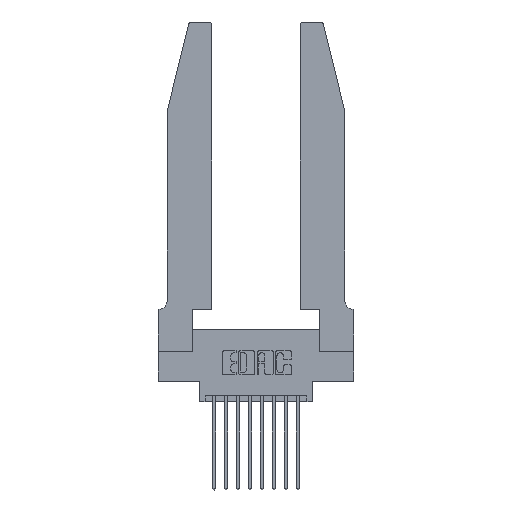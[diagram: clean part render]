
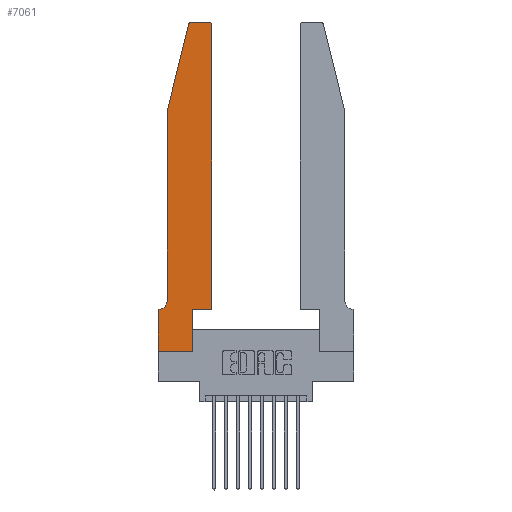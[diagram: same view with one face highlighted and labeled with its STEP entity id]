
A CAD part, top view. The second image highlights one B-rep face of the part: STEP entity #7061.
In plain terms, the highlighted planar face has unit normal (0, 0, 1).
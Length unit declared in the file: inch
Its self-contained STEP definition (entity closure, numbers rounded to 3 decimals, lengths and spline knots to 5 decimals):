
#55 = DIRECTION ( 'NONE',  ( 0., 1., 0. ) ) ;
#115 = VERTEX_POINT ( 'NONE', #11063 ) ;
#137 = VECTOR ( 'NONE', #9195, 39.37008 ) ;
#237 = LINE ( 'NONE', #2877, #425 ) ;
#254 = VERTEX_POINT ( 'NONE', #6310 ) ;
#397 = DIRECTION ( 'NONE',  ( 1., 0., 0. ) ) ;
#425 = VECTOR ( 'NONE', #13838, 39.37008 ) ;
#460 = VECTOR ( 'NONE', #7945, 39.37008 ) ;
#1157 = EDGE_CURVE ( 'NONE', #11795, #1531, #6339, .T. ) ;
#1382 = AXIS2_PLACEMENT_3D ( 'NONE', #1407, #3936, #6292 ) ;
#1407 = CARTESIAN_POINT ( 'NONE',  ( 0.0055, 0.42, 0.37 ) ) ;
#1531 = VERTEX_POINT ( 'NONE', #13340 ) ;
#1560 = DIRECTION ( 'NONE',  ( 0., 0., 1. ) ) ;
#1783 = LINE ( 'NONE', #11707, #460 ) ;
#1926 = CARTESIAN_POINT ( 'NONE',  ( 0.0755, 2., 0.37 ) ) ;
#2035 = CIRCLE ( 'NONE', #1382, 0.07 ) ;
#2506 = ORIENTED_EDGE ( 'NONE', *, *, #3610, .T. ) ;
#2720 = LINE ( 'NONE', #12124, #10547 ) ;
#2877 = CARTESIAN_POINT ( 'NONE',  ( 0.4505, 0.35, 0.37 ) ) ;
#3466 = LINE ( 'NONE', #9100, #14325 ) ;
#3610 = EDGE_CURVE ( 'NONE', #4110, #3991, #11367, .T. ) ;
#3641 = DIRECTION ( 'NONE',  ( 0., 1., 0. ) ) ;
#3936 = DIRECTION ( 'NONE',  ( 0., 0., -1. ) ) ;
#3991 = VERTEX_POINT ( 'NONE', #4832 ) ;
#4051 = VERTEX_POINT ( 'NONE', #15708 ) ;
#4110 = VERTEX_POINT ( 'NONE', #13651 ) ;
#4287 = ORIENTED_EDGE ( 'NONE', *, *, #9130, .T. ) ;
#4391 = LINE ( 'NONE', #13379, #8354 ) ;
#4583 = CARTESIAN_POINT ( 'NONE',  ( 0.4505, 0.35, 0.37 ) ) ;
#4595 = CARTESIAN_POINT ( 'NONE',  ( 0.0755, 2., 0.37 ) ) ;
#4832 = CARTESIAN_POINT ( 'NONE',  ( 0., 0., 0.37 ) ) ;
#4838 = ORIENTED_EDGE ( 'NONE', *, *, #13740, .T. ) ;
#5462 = VERTEX_POINT ( 'NONE', #14276 ) ;
#5578 = CARTESIAN_POINT ( 'NONE',  ( 0.25487, 2.72718, 0.37 ) ) ;
#5922 = VERTEX_POINT ( 'NONE', #12003 ) ;
#6208 = ORIENTED_EDGE ( 'NONE', *, *, #11518, .T. ) ;
#6292 = DIRECTION ( 'NONE',  ( -1., 0., 0. ) ) ;
#6310 = CARTESIAN_POINT ( 'NONE',  ( 0.2865, 0., 0.37 ) ) ;
#6339 = CIRCLE ( 'NONE', #13452, 0.03 ) ;
#6708 = CARTESIAN_POINT ( 'NONE',  ( 0.4505, 2.72, 0.37 ) ) ;
#7061 = ADVANCED_FACE ( 'NONE', ( #10238 ), #12466, .T. ) ;
#7253 = VERTEX_POINT ( 'NONE', #5578 ) ;
#7313 = LINE ( 'NONE', #4595, #12444 ) ;
#7570 = EDGE_CURVE ( 'NONE', #4051, #5922, #2035, .T. ) ;
#7691 = DIRECTION ( 'NONE',  ( 1., 0., 0. ) ) ;
#7941 = CARTESIAN_POINT ( 'NONE',  ( 0., 0., 0.37 ) ) ;
#7945 = DIRECTION ( 'NONE',  ( -1., 0., 0. ) ) ;
#8354 = VECTOR ( 'NONE', #8436, 39.37008 ) ;
#8436 = DIRECTION ( 'NONE',  ( -1., 0., 0. ) ) ;
#8528 = DIRECTION ( 'NONE',  ( 0., 0., 1. ) ) ;
#8828 = EDGE_CURVE ( 'NONE', #7253, #115, #12647, .T. ) ;
#8882 = EDGE_CURVE ( 'NONE', #5922, #4110, #1783, .T. ) ;
#9100 = CARTESIAN_POINT ( 'NONE',  ( 0.4505, 0.35, 0.37 ) ) ;
#9130 = EDGE_CURVE ( 'NONE', #254, #13071, #2720, .T. ) ;
#9151 = LINE ( 'NONE', #10193, #12000 ) ;
#9195 = DIRECTION ( 'NONE',  ( 0., -1., 0. ) ) ;
#9245 = ORIENTED_EDGE ( 'NONE', *, *, #10284, .T. ) ;
#9595 = DIRECTION ( 'NONE',  ( 1., 0., 0. ) ) ;
#9928 = ORIENTED_EDGE ( 'NONE', *, *, #8828, .T. ) ;
#9991 = EDGE_CURVE ( 'NONE', #13071, #11934, #237, .T. ) ;
#10193 = CARTESIAN_POINT ( 'NONE',  ( 0., 0., 0.37 ) ) ;
#10205 = AXIS2_PLACEMENT_3D ( 'NONE', #12532, #1560, #10293 ) ;
#10238 = FACE_OUTER_BOUND ( 'NONE', #11191, .T. ) ;
#10266 = ORIENTED_EDGE ( 'NONE', *, *, #8882, .T. ) ;
#10284 = EDGE_CURVE ( 'NONE', #5462, #7253, #14129, .T. ) ;
#10293 = DIRECTION ( 'NONE',  ( 1., 0., 0. ) ) ;
#10547 = VECTOR ( 'NONE', #55, 39.37008 ) ;
#10829 = CARTESIAN_POINT ( 'NONE',  ( 0.4205, 2.72, 0.37 ) ) ;
#11063 = CARTESIAN_POINT ( 'NONE',  ( 0.0755, 2., 0.37 ) ) ;
#11191 = EDGE_LOOP ( 'NONE', ( #4838, #9245, #9928, #15221, #13813, #10266, #2506, #14378, #4287, #13395, #6208, #13303 ) ) ;
#11367 = LINE ( 'NONE', #7941, #137 ) ;
#11371 = EDGE_CURVE ( 'NONE', #115, #4051, #7313, .T. ) ;
#11518 = EDGE_CURVE ( 'NONE', #11934, #11795, #3466, .T. ) ;
#11707 = CARTESIAN_POINT ( 'NONE',  ( 0.0755, 0.35, 0.37 ) ) ;
#11795 = VERTEX_POINT ( 'NONE', #6708 ) ;
#11934 = VERTEX_POINT ( 'NONE', #4583 ) ;
#12000 = VECTOR ( 'NONE', #397, 39.37008 ) ;
#12003 = CARTESIAN_POINT ( 'NONE',  ( 0.0055, 0.35, 0.37 ) ) ;
#12124 = CARTESIAN_POINT ( 'NONE',  ( 0.2865, 0.35, 0.37 ) ) ;
#12279 = EDGE_CURVE ( 'NONE', #3991, #254, #9151, .T. ) ;
#12444 = VECTOR ( 'NONE', #14359, 39.37008 ) ;
#12466 = PLANE ( 'NONE',  #15562 ) ;
#12532 = CARTESIAN_POINT ( 'NONE',  ( 0.284, 2.72, 0.37 ) ) ;
#12647 = LINE ( 'NONE', #1926, #15324 ) ;
#13071 = VERTEX_POINT ( 'NONE', #13244 ) ;
#13244 = CARTESIAN_POINT ( 'NONE',  ( 0.2865, 0.35, 0.37 ) ) ;
#13303 = ORIENTED_EDGE ( 'NONE', *, *, #1157, .T. ) ;
#13340 = CARTESIAN_POINT ( 'NONE',  ( 0.4205, 2.75, 0.37 ) ) ;
#13379 = CARTESIAN_POINT ( 'NONE',  ( 0.2605, 2.75, 0.37 ) ) ;
#13395 = ORIENTED_EDGE ( 'NONE', *, *, #9991, .T. ) ;
#13452 = AXIS2_PLACEMENT_3D ( 'NONE', #10829, #8528, #9595 ) ;
#13651 = CARTESIAN_POINT ( 'NONE',  ( 0., 0.35, 0.37 ) ) ;
#13740 = EDGE_CURVE ( 'NONE', #1531, #5462, #4391, .T. ) ;
#13813 = ORIENTED_EDGE ( 'NONE', *, *, #7570, .T. ) ;
#13838 = DIRECTION ( 'NONE',  ( 1., 0., 0. ) ) ;
#14129 = CIRCLE ( 'NONE', #10205, 0.03 ) ;
#14276 = CARTESIAN_POINT ( 'NONE',  ( 0.284, 2.75, 0.37 ) ) ;
#14325 = VECTOR ( 'NONE', #3641, 39.37008 ) ;
#14359 = DIRECTION ( 'NONE',  ( 0., -1., 0. ) ) ;
#14378 = ORIENTED_EDGE ( 'NONE', *, *, #12279, .T. ) ;
#14811 = CARTESIAN_POINT ( 'NONE',  ( 0., 0.35, 0.37 ) ) ;
#14965 = DIRECTION ( 'NONE',  ( 0., 0., 1. ) ) ;
#15221 = ORIENTED_EDGE ( 'NONE', *, *, #11371, .T. ) ;
#15324 = VECTOR ( 'NONE', #15342, 39.37008 ) ;
#15342 = DIRECTION ( 'NONE',  ( -0.239, -0.971, 0. ) ) ;
#15562 = AXIS2_PLACEMENT_3D ( 'NONE', #14811, #14965, #7691 ) ;
#15708 = CARTESIAN_POINT ( 'NONE',  ( 0.0755, 0.42, 0.37 ) ) ;
